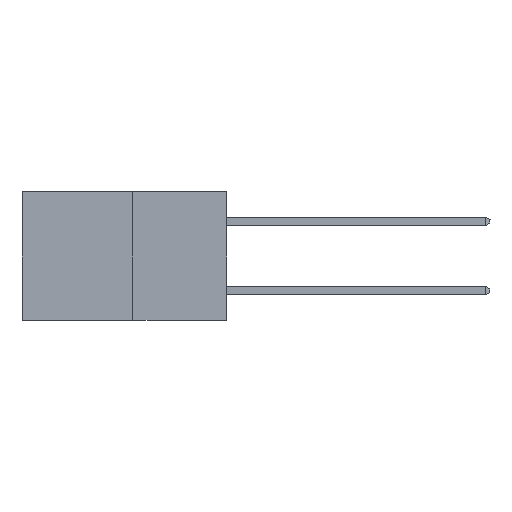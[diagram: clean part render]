
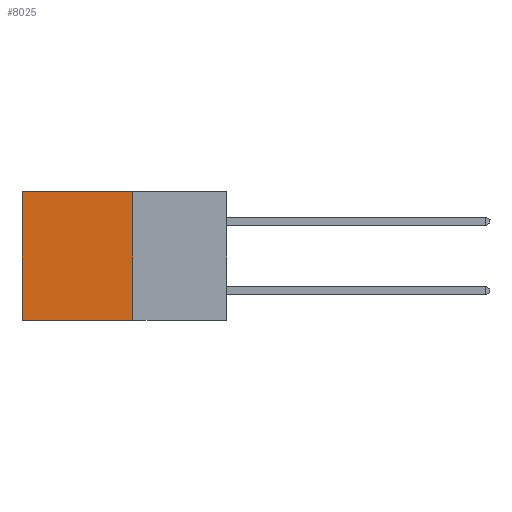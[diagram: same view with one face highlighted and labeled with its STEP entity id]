
A CAD part, left-side view. The second image highlights one B-rep face of the part: STEP entity #8025.
In plain terms, the highlighted planar face has unit normal (-1, 0, 0).
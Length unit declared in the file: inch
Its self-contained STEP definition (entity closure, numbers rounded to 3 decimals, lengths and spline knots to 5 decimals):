
#1514 = LINE ( 'NONE', #2387, #24369 ) ;
#2225 = VERTEX_POINT ( 'NONE', #16118 ) ;
#2387 = CARTESIAN_POINT ( 'NONE',  ( 0.277, 0.27, -0.37 ) ) ;
#3442 = CARTESIAN_POINT ( 'NONE',  ( 0.277, 0.59, -0.37 ) ) ;
#3444 = LINE ( 'NONE', #3442, #10020 ) ;
#4051 = ORIENTED_EDGE ( 'NONE', *, *, #18755, .F. ) ;
#5684 = DIRECTION ( 'NONE',  ( 0., 0., -1. ) ) ;
#5928 = CARTESIAN_POINT ( 'NONE',  ( 0.277, 0.27, -0.37 ) ) ;
#5946 = VECTOR ( 'NONE', #10348, 39.37008 ) ;
#6197 = VECTOR ( 'NONE', #21007, 39.37008 ) ;
#8025 = ADVANCED_FACE ( 'NONE', ( #18087 ), #26513, .F. ) ;
#8732 = CARTESIAN_POINT ( 'NONE',  ( 0.277, 0.59, 0. ) ) ;
#8771 = EDGE_LOOP ( 'NONE', ( #22453, #11086, #4051, #9405 ) ) ;
#9405 = ORIENTED_EDGE ( 'NONE', *, *, #9412, .T. ) ;
#9412 = EDGE_CURVE ( 'NONE', #10636, #16260, #23854, .T. ) ;
#10020 = VECTOR ( 'NONE', #5684, 39.37008 ) ;
#10198 = CARTESIAN_POINT ( 'NONE',  ( 0.277, 0.59, -0.37 ) ) ;
#10348 = DIRECTION ( 'NONE',  ( 0., 0., -1. ) ) ;
#10636 = VERTEX_POINT ( 'NONE', #16185 ) ;
#10815 = EDGE_CURVE ( 'NONE', #16260, #19884, #3444, .T. ) ;
#11086 = ORIENTED_EDGE ( 'NONE', *, *, #24143, .F. ) ;
#11814 = LINE ( 'NONE', #5928, #5946 ) ;
#12118 = AXIS2_PLACEMENT_3D ( 'NONE', #27325, #26458, #26423 ) ;
#15671 = DIRECTION ( 'NONE',  ( 0., 1., 0. ) ) ;
#16118 = CARTESIAN_POINT ( 'NONE',  ( 0.277, 0.27, -0.37 ) ) ;
#16185 = CARTESIAN_POINT ( 'NONE',  ( 0.277, 0.27, 0. ) ) ;
#16260 = VERTEX_POINT ( 'NONE', #8732 ) ;
#16527 = CARTESIAN_POINT ( 'NONE',  ( 0.277, 0.27, 0. ) ) ;
#18087 = FACE_OUTER_BOUND ( 'NONE', #8771, .T. ) ;
#18755 = EDGE_CURVE ( 'NONE', #10636, #2225, #11814, .T. ) ;
#19884 = VERTEX_POINT ( 'NONE', #10198 ) ;
#21007 = DIRECTION ( 'NONE',  ( 0., 1., 0. ) ) ;
#22453 = ORIENTED_EDGE ( 'NONE', *, *, #10815, .T. ) ;
#23854 = LINE ( 'NONE', #16527, #6197 ) ;
#24143 = EDGE_CURVE ( 'NONE', #2225, #19884, #1514, .T. ) ;
#24369 = VECTOR ( 'NONE', #15671, 39.37008 ) ;
#26423 = DIRECTION ( 'NONE',  ( 0., 0., -1. ) ) ;
#26458 = DIRECTION ( 'NONE',  ( 1., 0., 0. ) ) ;
#26513 = PLANE ( 'NONE',  #12118 ) ;
#27325 = CARTESIAN_POINT ( 'NONE',  ( 0.277, 0.27, -0.37 ) ) ;
